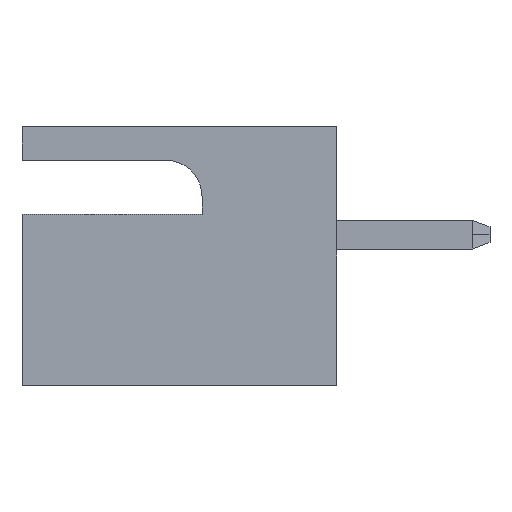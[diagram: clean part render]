
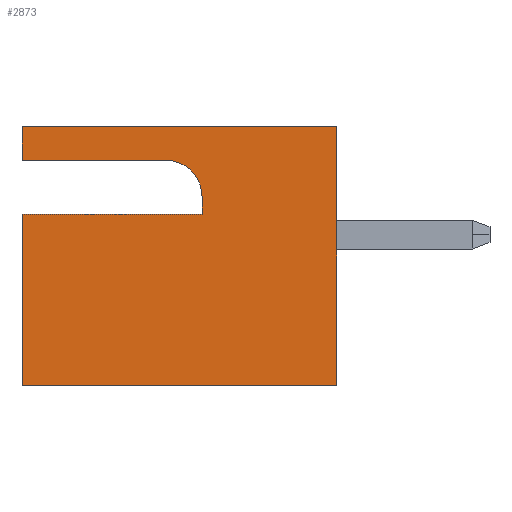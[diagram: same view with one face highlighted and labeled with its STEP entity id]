
A CAD part, left-side view. The second image highlights one B-rep face of the part: STEP entity #2873.
In plain terms, the highlighted planar face has unit normal (-1, 0, 0).
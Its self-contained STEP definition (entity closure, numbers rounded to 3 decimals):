
#37 = EDGE_CURVE ( 'NONE', #1733, #1739, #246, .T. ) ;
#86 = ORIENTED_EDGE ( 'NONE', *, *, #879, .T. ) ;
#206 = DIRECTION ( 'NONE',  ( 0., 0., -1. ) ) ;
#224 = CARTESIAN_POINT ( 'NONE',  ( -8.75, 7., -2.875 ) ) ;
#240 = CARTESIAN_POINT ( 'NONE',  ( -8.75, 0., -2.875 ) ) ;
#246 = LINE ( 'NONE', #224, #2335 ) ;
#265 = VECTOR ( 'NONE', #1776, 1000. ) ;
#331 = CARTESIAN_POINT ( 'NONE',  ( -8.75, 3.8, 2.125 ) ) ;
#342 = DIRECTION ( 'NONE',  ( 0., -1., 0. ) ) ;
#400 = CARTESIAN_POINT ( 'NONE',  ( -8.75, 7., -2.875 ) ) ;
#417 = EDGE_CURVE ( 'NONE', #1813, #1608, #1703, .T. ) ;
#480 = ORIENTED_EDGE ( 'NONE', *, *, #3870, .F. ) ;
#557 = CARTESIAN_POINT ( 'NONE',  ( -8.75, 3., 0.925 ) ) ;
#639 = PLANE ( 'NONE',  #3685 ) ;
#720 = VERTEX_POINT ( 'NONE', #2375 ) ;
#805 = EDGE_LOOP ( 'NONE', ( #3715, #3007, #891, #3769, #3081, #3223, #2679, #86, #480 ) ) ;
#879 = EDGE_CURVE ( 'NONE', #2552, #2476, #2823, .T. ) ;
#891 = ORIENTED_EDGE ( 'NONE', *, *, #417, .T. ) ;
#906 = DIRECTION ( 'NONE',  ( 0., 1., 0. ) ) ;
#938 = VERTEX_POINT ( 'NONE', #557 ) ;
#1039 = CARTESIAN_POINT ( 'NONE',  ( -8.75, 0., 2.875 ) ) ;
#1143 = CARTESIAN_POINT ( 'NONE',  ( -8.75, 7., 2.125 ) ) ;
#1198 = DIRECTION ( 'NONE',  ( 1., 0., 0. ) ) ;
#1266 = EDGE_CURVE ( 'NONE', #938, #720, #2174, .T. ) ;
#1319 = VECTOR ( 'NONE', #342, 1000. ) ;
#1334 = DIRECTION ( 'NONE',  ( 1., 0., 0. ) ) ;
#1456 = DIRECTION ( 'NONE',  ( 0., -1., 0. ) ) ;
#1486 = DIRECTION ( 'NONE',  ( 0., 0., 1. ) ) ;
#1557 = CARTESIAN_POINT ( 'NONE',  ( -8.75, 3.8, 1.325 ) ) ;
#1562 = CARTESIAN_POINT ( 'NONE',  ( -8.75, 7., 0.925 ) ) ;
#1599 = FACE_OUTER_BOUND ( 'NONE', #805, .T. ) ;
#1608 = VERTEX_POINT ( 'NONE', #3748 ) ;
#1703 = CIRCLE ( 'NONE', #3319, 0.8 ) ;
#1733 = VERTEX_POINT ( 'NONE', #2433 ) ;
#1739 = VERTEX_POINT ( 'NONE', #2542 ) ;
#1776 = DIRECTION ( 'NONE',  ( 0., -1., 0. ) ) ;
#1813 = VERTEX_POINT ( 'NONE', #331 ) ;
#1821 = DIRECTION ( 'NONE',  ( 0., 0., 1. ) ) ;
#1833 = DIRECTION ( 'NONE',  ( 0., 0., 1. ) ) ;
#1931 = CARTESIAN_POINT ( 'NONE',  ( -8.75, 7., -2.875 ) ) ;
#2022 = CARTESIAN_POINT ( 'NONE',  ( -8.75, 7., 2.875 ) ) ;
#2152 = LINE ( 'NONE', #3787, #3575 ) ;
#2174 = LINE ( 'NONE', #1562, #2446 ) ;
#2335 = VECTOR ( 'NONE', #1833, 1000. ) ;
#2375 = CARTESIAN_POINT ( 'NONE',  ( -8.75, 7., 0.925 ) ) ;
#2411 = LINE ( 'NONE', #1143, #265 ) ;
#2413 = VECTOR ( 'NONE', #1821, 1000. ) ;
#2433 = CARTESIAN_POINT ( 'NONE',  ( -8.75, 7., 2.125 ) ) ;
#2446 = VECTOR ( 'NONE', #906, 1000. ) ;
#2461 = CARTESIAN_POINT ( 'NONE',  ( -8.75, 7., -2.875 ) ) ;
#2476 = VERTEX_POINT ( 'NONE', #1039 ) ;
#2508 = LINE ( 'NONE', #3224, #1319 ) ;
#2542 = CARTESIAN_POINT ( 'NONE',  ( -8.75, 7., 2.875 ) ) ;
#2552 = VERTEX_POINT ( 'NONE', #240 ) ;
#2662 = LINE ( 'NONE', #2022, #4119 ) ;
#2679 = ORIENTED_EDGE ( 'NONE', *, *, #2782, .T. ) ;
#2782 = EDGE_CURVE ( 'NONE', #2897, #2552, #2508, .T. ) ;
#2823 = LINE ( 'NONE', #3116, #3128 ) ;
#2873 = ADVANCED_FACE ( 'NONE', ( #1599 ), #639, .F. ) ;
#2897 = VERTEX_POINT ( 'NONE', #400 ) ;
#3007 = ORIENTED_EDGE ( 'NONE', *, *, #3833, .T. ) ;
#3070 = EDGE_CURVE ( 'NONE', #2897, #720, #3710, .T. ) ;
#3081 = ORIENTED_EDGE ( 'NONE', *, *, #1266, .T. ) ;
#3099 = DIRECTION ( 'NONE',  ( 0., 0., -1. ) ) ;
#3116 = CARTESIAN_POINT ( 'NONE',  ( -8.75, 0., -2.875 ) ) ;
#3128 = VECTOR ( 'NONE', #1486, 1000. ) ;
#3223 = ORIENTED_EDGE ( 'NONE', *, *, #3070, .F. ) ;
#3224 = CARTESIAN_POINT ( 'NONE',  ( -8.75, 7., -2.875 ) ) ;
#3319 = AXIS2_PLACEMENT_3D ( 'NONE', #1557, #1198, #3099 ) ;
#3575 = VECTOR ( 'NONE', #206, 1000. ) ;
#3685 = AXIS2_PLACEMENT_3D ( 'NONE', #1931, #1334, #3921 ) ;
#3710 = LINE ( 'NONE', #2461, #2413 ) ;
#3715 = ORIENTED_EDGE ( 'NONE', *, *, #37, .F. ) ;
#3748 = CARTESIAN_POINT ( 'NONE',  ( -8.75, 3., 1.325 ) ) ;
#3769 = ORIENTED_EDGE ( 'NONE', *, *, #3976, .T. ) ;
#3787 = CARTESIAN_POINT ( 'NONE',  ( -8.75, 3., 1.325 ) ) ;
#3833 = EDGE_CURVE ( 'NONE', #1733, #1813, #2411, .T. ) ;
#3870 = EDGE_CURVE ( 'NONE', #1739, #2476, #2662, .T. ) ;
#3921 = DIRECTION ( 'NONE',  ( 0., 0., -1. ) ) ;
#3976 = EDGE_CURVE ( 'NONE', #1608, #938, #2152, .T. ) ;
#4119 = VECTOR ( 'NONE', #1456, 1000. ) ;
